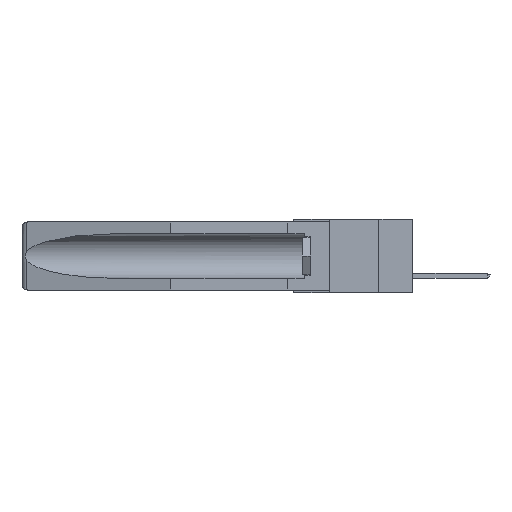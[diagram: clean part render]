
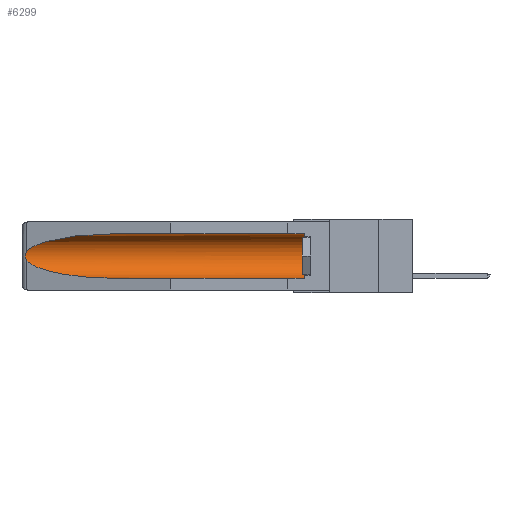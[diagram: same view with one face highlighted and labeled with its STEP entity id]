
A CAD part, left-side view. The second image highlights one B-rep face of the part: STEP entity #6299.
In plain terms, the highlighted cylindrical face has radius 2.857 mm (diameter 5.715 mm), a partial arc.
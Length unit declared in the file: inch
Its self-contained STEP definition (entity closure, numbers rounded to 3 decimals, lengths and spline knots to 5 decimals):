
#388 = CARTESIAN_POINT ( 'NONE',  ( 0.26537, 1.52718, -0.14972 ) ) ;
#691 = DIRECTION ( 'NONE',  ( 0., 1., 0. ) ) ;
#908 = CARTESIAN_POINT ( 'NONE',  ( 0.155, 1.07973, -0.284 ) ) ;
#1114 = CARTESIAN_POINT ( 'NONE',  ( 0.26654, 1.53092, -0.15636 ) ) ;
#1955 = CARTESIAN_POINT ( 'NONE',  ( 0.155, 0.126, -0.059 ) ) ;
#3190 = DIRECTION ( 'NONE',  ( 0., 1., 0. ) ) ;
#3261 = CARTESIAN_POINT ( 'NONE',  ( 0.155, 1.07973, -0.059 ) ) ;
#3322 = LINE ( 'NONE', #21178, #8996 ) ;
#3492 = AXIS2_PLACEMENT_3D ( 'NONE', #16527, #12870, #22455 ) ;
#4571 = VERTEX_POINT ( 'NONE', #12704 ) ;
#5228 = CARTESIAN_POINT ( 'NONE',  ( 0.2673, 1.53269, -0.17917 ) ) ;
#5522 = CARTESIAN_POINT ( 'NONE',  ( 0.155, 1.07973, -0.059 ) ) ;
#6299 = ADVANCED_FACE ( 'NONE', ( #20913 ), #20302, .F. ) ;
#7439 = CARTESIAN_POINT ( 'NONE',  ( 0.26537, 1.52718, -0.19328 ) ) ;
#7665 = VERTEX_POINT ( 'NONE', #23677 ) ;
#8087 = CARTESIAN_POINT ( 'NONE',  ( 0.26537, 1.52718, -0.14972 ) ) ;
#8607 = VERTEX_POINT ( 'NONE', #10396 ) ;
#8612 = CARTESIAN_POINT ( 'NONE',  ( 0.2673, 1.5327, -0.16383 ) ) ;
#8863 = EDGE_CURVE ( 'NONE', #4571, #17351, #21343, .T. ) ;
#8873 = EDGE_CURVE ( 'NONE', #8607, #4571, #23741, .T. ) ;
#8996 = VECTOR ( 'NONE', #13665, 39.37008 ) ;
#9101 =( BOUNDED_CURVE ( )  B_SPLINE_CURVE ( 3, ( #5522, #18873, #11771, #8087 ),
 .UNSPECIFIED., .F., .T. ) 
 B_SPLINE_CURVE_WITH_KNOTS ( ( 4, 4 ),
 ( 4.71239, 6.08839 ),
 .UNSPECIFIED. ) 
 CURVE ( )  GEOMETRIC_REPRESENTATION_ITEM ( )  RATIONAL_B_SPLINE_CURVE ( ( 1., 0.848, 0.848, 1. ) ) 
 REPRESENTATION_ITEM ( '' )  );
#9983 = VERTEX_POINT ( 'NONE', #3261 ) ;
#10055 = CARTESIAN_POINT ( 'NONE',  ( 0.2675, 1.53308, -0.16763 ) ) ;
#10237 = ORIENTED_EDGE ( 'NONE', *, *, #11815, .T. ) ;
#10396 = CARTESIAN_POINT ( 'NONE',  ( 0.26537, 1.52718, -0.14972 ) ) ;
#11771 = CARTESIAN_POINT ( 'NONE',  ( 0.25451, 1.48313, -0.09465 ) ) ;
#11815 = EDGE_CURVE ( 'NONE', #15762, #9983, #16604, .T. ) ;
#12199 = EDGE_CURVE ( 'NONE', #7665, #17351, #3322, .T. ) ;
#12704 = CARTESIAN_POINT ( 'NONE',  ( 0.26537, 1.52718, -0.19328 ) ) ;
#12870 = DIRECTION ( 'NONE',  ( 0., -1., 0. ) ) ;
#13163 = AXIS2_PLACEMENT_3D ( 'NONE', #17671, #691, #19072 ) ;
#13665 = DIRECTION ( 'NONE',  ( 0., 1., 0. ) ) ;
#13732 = EDGE_CURVE ( 'NONE', #7665, #15762, #23497, .T. ) ;
#13741 = ORIENTED_EDGE ( 'NONE', *, *, #15836, .T. ) ;
#15334 = ORIENTED_EDGE ( 'NONE', *, *, #12199, .F. ) ;
#15418 = VECTOR ( 'NONE', #3190, 39.37008 ) ;
#15718 = CARTESIAN_POINT ( 'NONE',  ( 0.2675, 1.53308, -0.17534 ) ) ;
#15762 = VERTEX_POINT ( 'NONE', #1955 ) ;
#15836 = EDGE_CURVE ( 'NONE', #9983, #8607, #9101, .T. ) ;
#16040 = CARTESIAN_POINT ( 'NONE',  ( 0.21114, 1.30732, -0.284 ) ) ;
#16177 = ORIENTED_EDGE ( 'NONE', *, *, #13732, .T. ) ;
#16527 = CARTESIAN_POINT ( 'NONE',  ( 0.155, 0.126, -0.1715 ) ) ;
#16568 = ORIENTED_EDGE ( 'NONE', *, *, #8863, .T. ) ;
#16604 = LINE ( 'NONE', #16677, #15418 ) ;
#16677 = CARTESIAN_POINT ( 'NONE',  ( 0.155, -0.30754, -0.059 ) ) ;
#16909 = CARTESIAN_POINT ( 'NONE',  ( 0.26597, 1.5296, -0.19026 ) ) ;
#17351 = VERTEX_POINT ( 'NONE', #24341 ) ;
#17671 = CARTESIAN_POINT ( 'NONE',  ( 0.155, -0.30754, -0.1715 ) ) ;
#17890 = CARTESIAN_POINT ( 'NONE',  ( 0.25451, 1.48313, -0.24835 ) ) ;
#18705 = ORIENTED_EDGE ( 'NONE', *, *, #8873, .T. ) ;
#18873 = CARTESIAN_POINT ( 'NONE',  ( 0.21114, 1.30732, -0.059 ) ) ;
#18992 = CARTESIAN_POINT ( 'NONE',  ( 0.26597, 1.52961, -0.15275 ) ) ;
#19072 = DIRECTION ( 'NONE',  ( 0., 0., 1. ) ) ;
#20302 = CYLINDRICAL_SURFACE ( 'NONE', #13163, 0.1125 ) ;
#20836 = CARTESIAN_POINT ( 'NONE',  ( 0.26655, 1.53094, -0.18657 ) ) ;
#20913 = FACE_OUTER_BOUND ( 'NONE', #22236, .T. ) ;
#21178 = CARTESIAN_POINT ( 'NONE',  ( 0.155, -0.30754, -0.284 ) ) ;
#21343 =( BOUNDED_CURVE ( )  B_SPLINE_CURVE ( 3, ( #23682, #17890, #16040, #908 ),
 .UNSPECIFIED., .F., .F. ) 
 B_SPLINE_CURVE_WITH_KNOTS ( ( 4, 4 ),
 ( 0.1948, 1.5708 ),
 .UNSPECIFIED. ) 
 CURVE ( )  GEOMETRIC_REPRESENTATION_ITEM ( )  RATIONAL_B_SPLINE_CURVE ( ( 1., 0.848, 0.848, 1. ) ) 
 REPRESENTATION_ITEM ( '' )  );
#22236 = EDGE_LOOP ( 'NONE', ( #13741, #18705, #16568, #15334, #16177, #10237 ) ) ;
#22455 = DIRECTION ( 'NONE',  ( 0., 0., 1. ) ) ;
#23497 = CIRCLE ( 'NONE', #3492, 0.1125 ) ;
#23677 = CARTESIAN_POINT ( 'NONE',  ( 0.155, 0.126, -0.284 ) ) ;
#23682 = CARTESIAN_POINT ( 'NONE',  ( 0.26537, 1.52718, -0.19328 ) ) ;
#23741 = B_SPLINE_CURVE_WITH_KNOTS ( 'NONE', 3,
 ( #388, #18992, #1114, #8612, #10055, #15718, #5228, #20836, #16909, #7439 ),
 .UNSPECIFIED., .F., .F.,
 ( 4, 2, 2, 2, 4 ),
 ( 0., 0.00029, 0.00058, 0.00087, 0.00117 ),
 .UNSPECIFIED. ) ;
#24341 = CARTESIAN_POINT ( 'NONE',  ( 0.155, 1.07973, -0.284 ) ) ;
